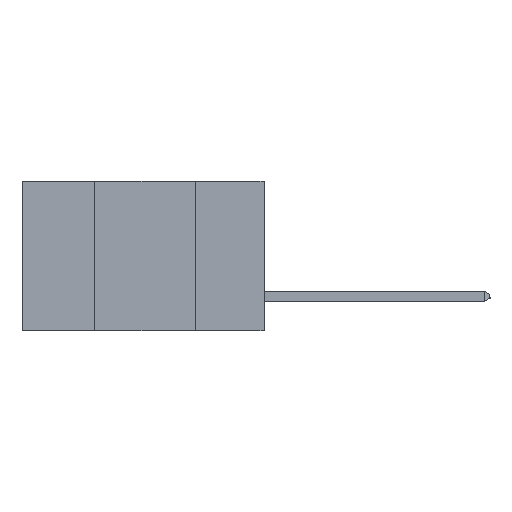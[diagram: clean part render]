
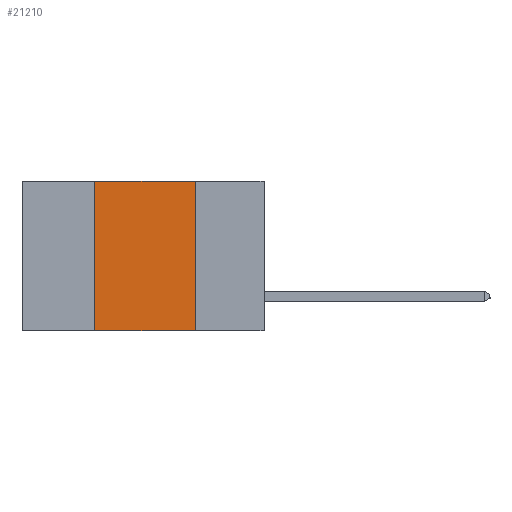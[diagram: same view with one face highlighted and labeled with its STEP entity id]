
A CAD part, left-side view. The second image highlights one B-rep face of the part: STEP entity #21210.
In plain terms, the highlighted planar face has unit normal (-1, 0, 0).
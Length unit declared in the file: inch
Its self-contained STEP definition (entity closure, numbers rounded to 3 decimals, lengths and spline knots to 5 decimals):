
#351 = ORIENTED_EDGE ( 'NONE', *, *, #14479, .T. ) ;
#994 = VECTOR ( 'NONE', #14296, 39.37008 ) ;
#1095 = ORIENTED_EDGE ( 'NONE', *, *, #17614, .F. ) ;
#3183 = ORIENTED_EDGE ( 'NONE', *, *, #21990, .F. ) ;
#3864 = VECTOR ( 'NONE', #31574, 39.37008 ) ;
#5623 = CARTESIAN_POINT ( 'NONE',  ( 0., 0.6, -0.37 ) ) ;
#5641 = FACE_OUTER_BOUND ( 'NONE', #15061, .T. ) ;
#6389 = ORIENTED_EDGE ( 'NONE', *, *, #7233, .F. ) ;
#6827 = CARTESIAN_POINT ( 'NONE',  ( 0., 0.6, 0. ) ) ;
#6853 = VERTEX_POINT ( 'NONE', #7572 ) ;
#7233 = EDGE_CURVE ( 'NONE', #10259, #25926, #23578, .T. ) ;
#7553 = LINE ( 'NONE', #6827, #994 ) ;
#7572 = CARTESIAN_POINT ( 'NONE',  ( 0., 0.17, 0. ) ) ;
#8303 = CARTESIAN_POINT ( 'NONE',  ( 0., 0.17, 0. ) ) ;
#8557 = VECTOR ( 'NONE', #27875, 39.37008 ) ;
#10259 = VERTEX_POINT ( 'NONE', #23933 ) ;
#11397 = VECTOR ( 'NONE', #23105, 39.37008 ) ;
#11614 = AXIS2_PLACEMENT_3D ( 'NONE', #28473, #13687, #30885 ) ;
#13687 = DIRECTION ( 'NONE',  ( 1., 0., 0. ) ) ;
#14296 = DIRECTION ( 'NONE',  ( 0., -1., 0. ) ) ;
#14479 = EDGE_CURVE ( 'NONE', #10259, #18311, #21688, .T. ) ;
#15061 = EDGE_LOOP ( 'NONE', ( #1095, #3183, #6389, #351 ) ) ;
#17614 = EDGE_CURVE ( 'NONE', #6853, #18311, #24570, .T. ) ;
#18311 = VERTEX_POINT ( 'NONE', #25871 ) ;
#21210 = ADVANCED_FACE ( 'NONE', ( #5641 ), #26004, .F. ) ;
#21688 = LINE ( 'NONE', #5623, #8557 ) ;
#21990 = EDGE_CURVE ( 'NONE', #25926, #6853, #7553, .T. ) ;
#23105 = DIRECTION ( 'NONE',  ( 0., 0., -1. ) ) ;
#23578 = LINE ( 'NONE', #29134, #3864 ) ;
#23933 = CARTESIAN_POINT ( 'NONE',  ( 0., 0.42, -0.37 ) ) ;
#24570 = LINE ( 'NONE', #8303, #11397 ) ;
#25871 = CARTESIAN_POINT ( 'NONE',  ( 0., 0.17, -0.37 ) ) ;
#25926 = VERTEX_POINT ( 'NONE', #26224 ) ;
#26004 = PLANE ( 'NONE',  #11614 ) ;
#26224 = CARTESIAN_POINT ( 'NONE',  ( 0., 0.42, 0. ) ) ;
#27875 = DIRECTION ( 'NONE',  ( 0., -1., 0. ) ) ;
#28473 = CARTESIAN_POINT ( 'NONE',  ( 0., 0.6, 0. ) ) ;
#29134 = CARTESIAN_POINT ( 'NONE',  ( 0., 0.42, 0. ) ) ;
#30885 = DIRECTION ( 'NONE',  ( 0., 0., -1. ) ) ;
#31574 = DIRECTION ( 'NONE',  ( 0., 0., 1. ) ) ;
